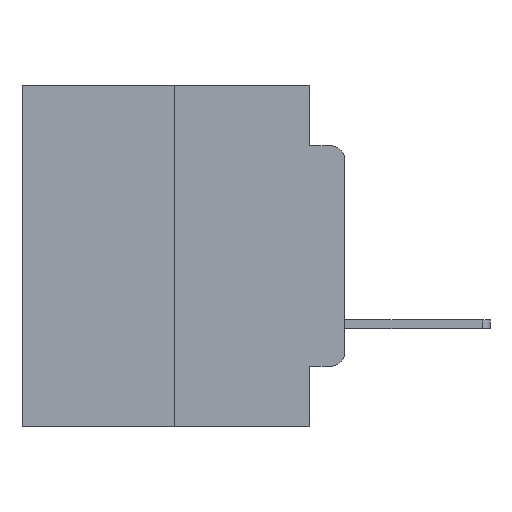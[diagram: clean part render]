
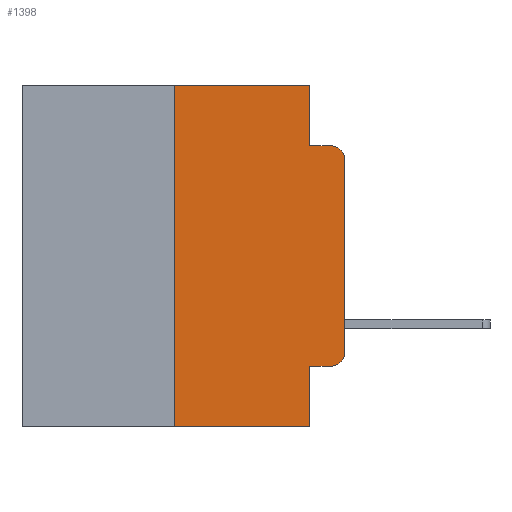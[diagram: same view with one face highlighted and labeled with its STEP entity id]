
A CAD part, left-side view. The second image highlights one B-rep face of the part: STEP entity #1398.
In plain terms, the highlighted planar face has unit normal (-1, 0, 0).
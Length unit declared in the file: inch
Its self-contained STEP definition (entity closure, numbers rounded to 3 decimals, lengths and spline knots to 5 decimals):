
#90 = DIRECTION ( 'NONE',  ( -1., 0., 0. ) ) ;
#667 = CIRCLE ( 'NONE', #8616, 0.02 ) ;
#1361 = DIRECTION ( 'NONE',  ( 0., -1., 0. ) ) ;
#1398 = ADVANCED_FACE ( 'NONE', ( #26274 ), #10116, .F. ) ;
#1545 = VERTEX_POINT ( 'NONE', #12796 ) ;
#1643 = CARTESIAN_POINT ( 'NONE',  ( 0., 0.473, 0. ) ) ;
#1730 = VECTOR ( 'NONE', #1361, 39.37008 ) ;
#3025 = LINE ( 'NONE', #22724, #24138 ) ;
#4599 = CARTESIAN_POINT ( 'NONE',  ( 0., 0., 0. ) ) ;
#5098 = EDGE_CURVE ( 'NONE', #5623, #8438, #16386, .T. ) ;
#5104 = LINE ( 'NONE', #4599, #26032 ) ;
#5376 = ORIENTED_EDGE ( 'NONE', *, *, #16146, .T. ) ;
#5623 = VERTEX_POINT ( 'NONE', #20592 ) ;
#5764 = EDGE_CURVE ( 'NONE', #1545, #16122, #5104, .T. ) ;
#6054 = DIRECTION ( 'NONE',  ( 0., -1., 0. ) ) ;
#6301 = EDGE_CURVE ( 'NONE', #14777, #5623, #3025, .T. ) ;
#6803 = LINE ( 'NONE', #7563, #16401 ) ;
#7253 = AXIS2_PLACEMENT_3D ( 'NONE', #1643, #12164, #26244 ) ;
#7377 = LINE ( 'NONE', #13816, #22903 ) ;
#7563 = CARTESIAN_POINT ( 'NONE',  ( 0., 0.051, 0. ) ) ;
#7598 = CARTESIAN_POINT ( 'NONE',  ( 0., 0., -0.1085 ) ) ;
#7662 = ORIENTED_EDGE ( 'NONE', *, *, #5098, .F. ) ;
#8257 = VERTEX_POINT ( 'NONE', #17510 ) ;
#8297 = ORIENTED_EDGE ( 'NONE', *, *, #12652, .T. ) ;
#8438 = VERTEX_POINT ( 'NONE', #26051 ) ;
#8616 = AXIS2_PLACEMENT_3D ( 'NONE', #12729, #90, #14780 ) ;
#10116 = PLANE ( 'NONE',  #7253 ) ;
#10590 = DIRECTION ( 'NONE',  ( 0., 0., 1. ) ) ;
#11005 = DIRECTION ( 'NONE',  ( 0., -1., 0. ) ) ;
#11154 = ORIENTED_EDGE ( 'NONE', *, *, #14524, .F. ) ;
#11472 = EDGE_LOOP ( 'NONE', ( #15313, #21318, #26584, #11154, #7662, #23801, #8297, #15010, #20393, #5376 ) ) ;
#11763 = DIRECTION ( 'NONE',  ( -1., 0., 0. ) ) ;
#11816 = CARTESIAN_POINT ( 'NONE',  ( 0., 0.473, -0.5 ) ) ;
#12164 = DIRECTION ( 'NONE',  ( 1., 0., 0. ) ) ;
#12634 = CARTESIAN_POINT ( 'NONE',  ( 0., 0.25, -0.5 ) ) ;
#12652 = EDGE_CURVE ( 'NONE', #14777, #21031, #12855, .T. ) ;
#12729 = CARTESIAN_POINT ( 'NONE',  ( 0., 0.02, -0.1085 ) ) ;
#12779 = VECTOR ( 'NONE', #13161, 39.37008 ) ;
#12796 = CARTESIAN_POINT ( 'NONE',  ( 0., 0., -0.3915 ) ) ;
#12855 = LINE ( 'NONE', #11816, #1730 ) ;
#13161 = DIRECTION ( 'NONE',  ( 0., -1., 0. ) ) ;
#13420 = LINE ( 'NONE', #21217, #12779 ) ;
#13816 = CARTESIAN_POINT ( 'NONE',  ( 0., 0.051, 0. ) ) ;
#14524 = EDGE_CURVE ( 'NONE', #8438, #8257, #7377, .T. ) ;
#14533 = CARTESIAN_POINT ( 'NONE',  ( 0., 0.02, -0.0885 ) ) ;
#14777 = VERTEX_POINT ( 'NONE', #12634 ) ;
#14780 = DIRECTION ( 'NONE',  ( 0., 0., -1. ) ) ;
#14932 = EDGE_CURVE ( 'NONE', #19477, #23124, #13420, .T. ) ;
#15010 = ORIENTED_EDGE ( 'NONE', *, *, #26398, .F. ) ;
#15154 = CARTESIAN_POINT ( 'NONE',  ( 0., 0.051, -0.4115 ) ) ;
#15313 = ORIENTED_EDGE ( 'NONE', *, *, #5764, .T. ) ;
#15509 = VECTOR ( 'NONE', #6054, 39.37008 ) ;
#15731 = VECTOR ( 'NONE', #11005, 39.37008 ) ;
#16122 = VERTEX_POINT ( 'NONE', #7598 ) ;
#16146 = EDGE_CURVE ( 'NONE', #23124, #1545, #26533, .T. ) ;
#16386 = LINE ( 'NONE', #21124, #15731 ) ;
#16401 = VECTOR ( 'NONE', #23750, 39.37008 ) ;
#17510 = CARTESIAN_POINT ( 'NONE',  ( 0., 0.051, -0.0885 ) ) ;
#19259 = VERTEX_POINT ( 'NONE', #14533 ) ;
#19477 = VERTEX_POINT ( 'NONE', #15154 ) ;
#19955 = DIRECTION ( 'NONE',  ( 0., 0., -1. ) ) ;
#20234 = CARTESIAN_POINT ( 'NONE',  ( 0., 0.051, -0.0885 ) ) ;
#20393 = ORIENTED_EDGE ( 'NONE', *, *, #14932, .T. ) ;
#20592 = CARTESIAN_POINT ( 'NONE',  ( 0., 0.25, 0. ) ) ;
#20927 = DIRECTION ( 'NONE',  ( 0., 0., 1. ) ) ;
#21031 = VERTEX_POINT ( 'NONE', #25378 ) ;
#21124 = CARTESIAN_POINT ( 'NONE',  ( 0., 0.473, 0. ) ) ;
#21217 = CARTESIAN_POINT ( 'NONE',  ( 0., 0.051, -0.4115 ) ) ;
#21300 = EDGE_CURVE ( 'NONE', #8257, #19259, #26158, .T. ) ;
#21318 = ORIENTED_EDGE ( 'NONE', *, *, #26612, .T. ) ;
#22724 = CARTESIAN_POINT ( 'NONE',  ( 0., 0.25, 0. ) ) ;
#22903 = VECTOR ( 'NONE', #19955, 39.37008 ) ;
#23124 = VERTEX_POINT ( 'NONE', #26300 ) ;
#23750 = DIRECTION ( 'NONE',  ( 0., 0., -1. ) ) ;
#23801 = ORIENTED_EDGE ( 'NONE', *, *, #6301, .F. ) ;
#23876 = CARTESIAN_POINT ( 'NONE',  ( 0., 0.02, -0.3915 ) ) ;
#23957 = AXIS2_PLACEMENT_3D ( 'NONE', #23876, #11763, #25869 ) ;
#24138 = VECTOR ( 'NONE', #10590, 39.37008 ) ;
#25378 = CARTESIAN_POINT ( 'NONE',  ( 0., 0.051, -0.5 ) ) ;
#25869 = DIRECTION ( 'NONE',  ( 0., 0., -1. ) ) ;
#26032 = VECTOR ( 'NONE', #20927, 39.37008 ) ;
#26051 = CARTESIAN_POINT ( 'NONE',  ( 0., 0.051, 0. ) ) ;
#26158 = LINE ( 'NONE', #20234, #15509 ) ;
#26244 = DIRECTION ( 'NONE',  ( 0., 0., -1. ) ) ;
#26274 = FACE_OUTER_BOUND ( 'NONE', #11472, .T. ) ;
#26300 = CARTESIAN_POINT ( 'NONE',  ( 0., 0.02, -0.4115 ) ) ;
#26398 = EDGE_CURVE ( 'NONE', #19477, #21031, #6803, .T. ) ;
#26533 = CIRCLE ( 'NONE', #23957, 0.02 ) ;
#26584 = ORIENTED_EDGE ( 'NONE', *, *, #21300, .F. ) ;
#26612 = EDGE_CURVE ( 'NONE', #16122, #19259, #667, .T. ) ;
